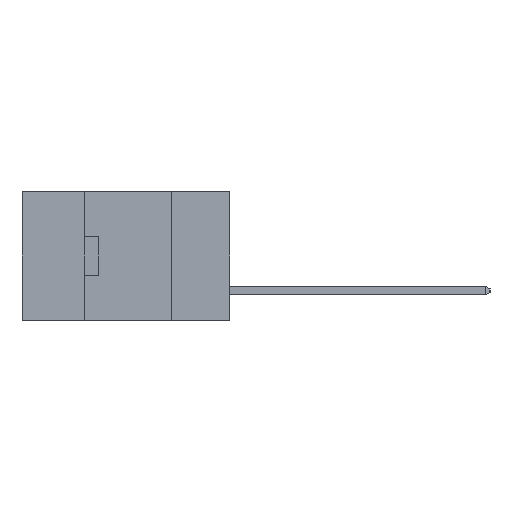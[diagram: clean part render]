
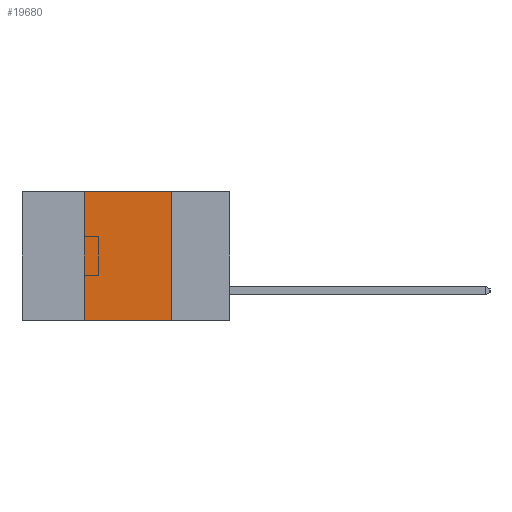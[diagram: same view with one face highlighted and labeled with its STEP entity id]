
A CAD part, left-side view. The second image highlights one B-rep face of the part: STEP entity #19680.
In plain terms, the highlighted planar face has unit normal (-1, 0, 0).
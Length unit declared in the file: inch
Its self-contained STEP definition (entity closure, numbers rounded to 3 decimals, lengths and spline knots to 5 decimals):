
#455 = LINE ( 'NONE', #25585, #21243 ) ;
#694 = DIRECTION ( 'NONE',  ( 0., -1., 0. ) ) ;
#787 = CARTESIAN_POINT ( 'NONE',  ( 0., 0.6, -0.37 ) ) ;
#1083 = VERTEX_POINT ( 'NONE', #23282 ) ;
#3631 = VECTOR ( 'NONE', #19149, 39.37008 ) ;
#3653 = EDGE_CURVE ( 'NONE', #6940, #11133, #19963, .T. ) ;
#3818 = EDGE_CURVE ( 'NONE', #1083, #17867, #455, .T. ) ;
#4542 = ORIENTED_EDGE ( 'NONE', *, *, #3818, .F. ) ;
#6940 = VERTEX_POINT ( 'NONE', #17698 ) ;
#7965 = ORIENTED_EDGE ( 'NONE', *, *, #3653, .T. ) ;
#9100 = FACE_OUTER_BOUND ( 'NONE', #13262, .T. ) ;
#9367 = ORIENTED_EDGE ( 'NONE', *, *, #23317, .F. ) ;
#9994 = VECTOR ( 'NONE', #11259, 39.37008 ) ;
#11042 = CARTESIAN_POINT ( 'NONE',  ( 0., 0.42, -0.37 ) ) ;
#11133 = VERTEX_POINT ( 'NONE', #14788 ) ;
#11259 = DIRECTION ( 'NONE',  ( 0., 0., -1. ) ) ;
#12531 = DIRECTION ( 'NONE',  ( 0., 0., -1. ) ) ;
#12705 = CARTESIAN_POINT ( 'NONE',  ( 0., 0.17, 0. ) ) ;
#13262 = EDGE_LOOP ( 'NONE', ( #25558, #4542, #9367, #7965 ) ) ;
#14004 = LINE ( 'NONE', #11042, #3631 ) ;
#14788 = CARTESIAN_POINT ( 'NONE',  ( 0., 0.17, -0.37 ) ) ;
#15933 = EDGE_CURVE ( 'NONE', #17867, #11133, #25403, .T. ) ;
#17698 = CARTESIAN_POINT ( 'NONE',  ( 0., 0.42, -0.37 ) ) ;
#17867 = VERTEX_POINT ( 'NONE', #12705 ) ;
#19149 = DIRECTION ( 'NONE',  ( 0., 0., 1. ) ) ;
#19316 = VECTOR ( 'NONE', #694, 39.37008 ) ;
#19680 = ADVANCED_FACE ( 'NONE', ( #9100 ), #22613, .F. ) ;
#19963 = LINE ( 'NONE', #787, #19316 ) ;
#20617 = CARTESIAN_POINT ( 'NONE',  ( 0., 0.6, 0. ) ) ;
#21243 = VECTOR ( 'NONE', #21622, 39.37008 ) ;
#21622 = DIRECTION ( 'NONE',  ( 0., -1., 0. ) ) ;
#22613 = PLANE ( 'NONE',  #25951 ) ;
#23282 = CARTESIAN_POINT ( 'NONE',  ( 0., 0.42, 0. ) ) ;
#23317 = EDGE_CURVE ( 'NONE', #6940, #1083, #14004, .T. ) ;
#23364 = CARTESIAN_POINT ( 'NONE',  ( 0., 0.17, -0.37 ) ) ;
#24544 = DIRECTION ( 'NONE',  ( 1., 0., 0. ) ) ;
#25403 = LINE ( 'NONE', #23364, #9994 ) ;
#25558 = ORIENTED_EDGE ( 'NONE', *, *, #15933, .F. ) ;
#25585 = CARTESIAN_POINT ( 'NONE',  ( 0., 0.6, 0. ) ) ;
#25951 = AXIS2_PLACEMENT_3D ( 'NONE', #20617, #24544, #12531 ) ;
